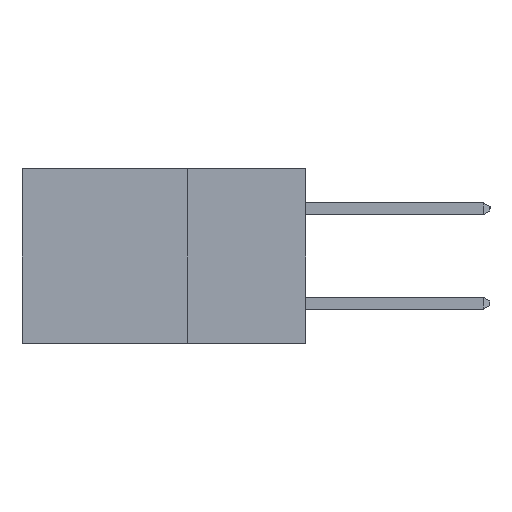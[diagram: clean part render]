
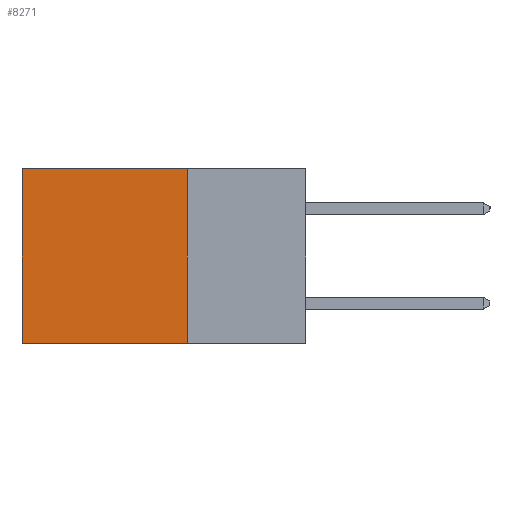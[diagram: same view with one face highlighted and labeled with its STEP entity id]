
A CAD part, left-side view. The second image highlights one B-rep face of the part: STEP entity #8271.
In plain terms, the highlighted planar face has unit normal (-1, 0, 0).
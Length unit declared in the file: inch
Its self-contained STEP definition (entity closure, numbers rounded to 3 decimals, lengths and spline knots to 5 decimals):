
#432 = EDGE_CURVE ( 'NONE', #5443, #11390, #3462, .T. ) ;
#1093 = CARTESIAN_POINT ( 'NONE',  ( 0.2615, 0.6, -0.37 ) ) ;
#1303 = VECTOR ( 'NONE', #6943, 39.37008 ) ;
#1819 = CARTESIAN_POINT ( 'NONE',  ( 0.2615, 0.25, -0.37 ) ) ;
#1867 = VECTOR ( 'NONE', #6356, 39.37008 ) ;
#2781 = LINE ( 'NONE', #8033, #1303 ) ;
#3094 = EDGE_CURVE ( 'NONE', #7453, #12934, #4271, .T. ) ;
#3462 = LINE ( 'NONE', #11325, #11114 ) ;
#4271 = LINE ( 'NONE', #9595, #1867 ) ;
#4759 = DIRECTION ( 'NONE',  ( 0., 0., -1. ) ) ;
#5136 = DIRECTION ( 'NONE',  ( 0., 0., -1. ) ) ;
#5443 = VERTEX_POINT ( 'NONE', #13217 ) ;
#5656 = ORIENTED_EDGE ( 'NONE', *, *, #11308, .T. ) ;
#5754 = CARTESIAN_POINT ( 'NONE',  ( 0.2615, 0.25, -0.37 ) ) ;
#6213 = DIRECTION ( 'NONE',  ( 1., 0., 0. ) ) ;
#6356 = DIRECTION ( 'NONE',  ( 0., 0., -1. ) ) ;
#6666 = CARTESIAN_POINT ( 'NONE',  ( 0.2615, 0.6, 0. ) ) ;
#6755 = LINE ( 'NONE', #5754, #12113 ) ;
#6943 = DIRECTION ( 'NONE',  ( 0., 1., 0. ) ) ;
#7285 = FACE_OUTER_BOUND ( 'NONE', #11407, .T. ) ;
#7453 = VERTEX_POINT ( 'NONE', #6666 ) ;
#8033 = CARTESIAN_POINT ( 'NONE',  ( 0.2615, 0.25, 0. ) ) ;
#8271 = ADVANCED_FACE ( 'NONE', ( #7285 ), #11692, .F. ) ;
#9248 = CARTESIAN_POINT ( 'NONE',  ( 0.2615, 0.25, -0.37 ) ) ;
#9595 = CARTESIAN_POINT ( 'NONE',  ( 0.2615, 0.6, -0.37 ) ) ;
#10638 = EDGE_CURVE ( 'NONE', #11390, #12934, #6755, .T. ) ;
#11114 = VECTOR ( 'NONE', #4759, 39.37008 ) ;
#11308 = EDGE_CURVE ( 'NONE', #5443, #7453, #2781, .T. ) ;
#11325 = CARTESIAN_POINT ( 'NONE',  ( 0.2615, 0.25, -0.37 ) ) ;
#11390 = VERTEX_POINT ( 'NONE', #9248 ) ;
#11407 = EDGE_LOOP ( 'NONE', ( #13352, #12813, #11409, #5656 ) ) ;
#11409 = ORIENTED_EDGE ( 'NONE', *, *, #432, .F. ) ;
#11692 = PLANE ( 'NONE',  #12967 ) ;
#12113 = VECTOR ( 'NONE', #13434, 39.37008 ) ;
#12813 = ORIENTED_EDGE ( 'NONE', *, *, #10638, .F. ) ;
#12934 = VERTEX_POINT ( 'NONE', #1093 ) ;
#12967 = AXIS2_PLACEMENT_3D ( 'NONE', #1819, #6213, #5136 ) ;
#13217 = CARTESIAN_POINT ( 'NONE',  ( 0.2615, 0.25, 0. ) ) ;
#13352 = ORIENTED_EDGE ( 'NONE', *, *, #3094, .T. ) ;
#13434 = DIRECTION ( 'NONE',  ( 0., 1., 0. ) ) ;
